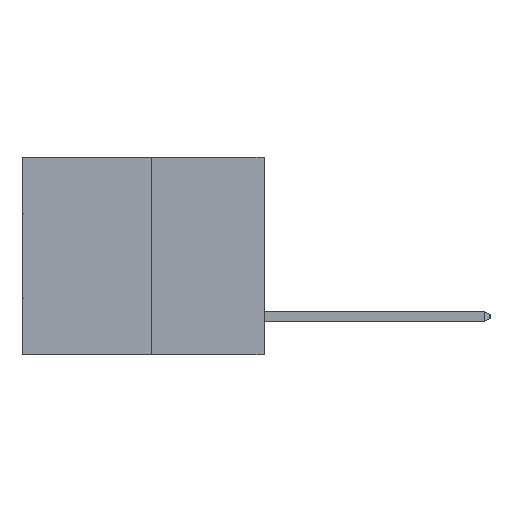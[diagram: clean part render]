
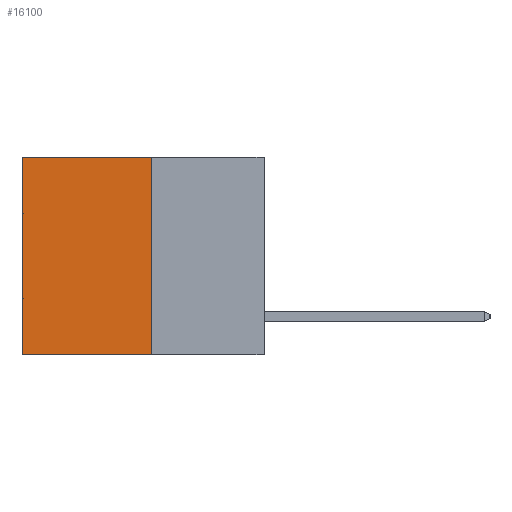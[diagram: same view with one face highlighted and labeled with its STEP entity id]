
A CAD part, left-side view. The second image highlights one B-rep face of the part: STEP entity #16100.
In plain terms, the highlighted planar face has unit normal (-1, 0, 0).
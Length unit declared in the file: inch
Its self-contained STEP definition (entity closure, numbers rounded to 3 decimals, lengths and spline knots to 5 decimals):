
#601 = CARTESIAN_POINT ( 'NONE',  ( 0.3165, 0.6, -0.49 ) ) ;
#1386 = CARTESIAN_POINT ( 'NONE',  ( 0.3165, 0.6, -0.49 ) ) ;
#1654 = ORIENTED_EDGE ( 'NONE', *, *, #6146, .F. ) ;
#3973 = ORIENTED_EDGE ( 'NONE', *, *, #23346, .T. ) ;
#5171 = CARTESIAN_POINT ( 'NONE',  ( 0.3165, 0.28, -0.49 ) ) ;
#5346 = DIRECTION ( 'NONE',  ( 1., 0., 0. ) ) ;
#6009 = EDGE_CURVE ( 'NONE', #11540, #22095, #23398, .T. ) ;
#6086 = CARTESIAN_POINT ( 'NONE',  ( 0.3165, 0.6, 0. ) ) ;
#6146 = EDGE_CURVE ( 'NONE', #7820, #22095, #13781, .T. ) ;
#6306 = CARTESIAN_POINT ( 'NONE',  ( 0.3165, 0.28, -0.49 ) ) ;
#7820 = VERTEX_POINT ( 'NONE', #5171 ) ;
#9064 = FACE_OUTER_BOUND ( 'NONE', #12457, .T. ) ;
#10021 = CARTESIAN_POINT ( 'NONE',  ( 0.3165, 0.28, 0. ) ) ;
#10143 = VECTOR ( 'NONE', #27080, 39.37008 ) ;
#10297 = DIRECTION ( 'NONE',  ( 0., 0., -1. ) ) ;
#11540 = VERTEX_POINT ( 'NONE', #6086 ) ;
#12457 = EDGE_LOOP ( 'NONE', ( #30422, #1654, #18782, #3973 ) ) ;
#13781 = LINE ( 'NONE', #21699, #14905 ) ;
#14905 = VECTOR ( 'NONE', #19558, 39.37008 ) ;
#16100 = ADVANCED_FACE ( 'NONE', ( #9064 ), #16846, .F. ) ;
#16790 = AXIS2_PLACEMENT_3D ( 'NONE', #24433, #5346, #24334 ) ;
#16846 = PLANE ( 'NONE',  #16790 ) ;
#16871 = VECTOR ( 'NONE', #10297, 39.37008 ) ;
#17256 = VERTEX_POINT ( 'NONE', #10021 ) ;
#18273 = VECTOR ( 'NONE', #28182, 39.37008 ) ;
#18782 = ORIENTED_EDGE ( 'NONE', *, *, #30556, .F. ) ;
#19558 = DIRECTION ( 'NONE',  ( 0., 1., 0. ) ) ;
#19794 = LINE ( 'NONE', #29363, #10143 ) ;
#21699 = CARTESIAN_POINT ( 'NONE',  ( 0.3165, 0.28, -0.49 ) ) ;
#22095 = VERTEX_POINT ( 'NONE', #601 ) ;
#23346 = EDGE_CURVE ( 'NONE', #17256, #11540, #19794, .T. ) ;
#23398 = LINE ( 'NONE', #1386, #16871 ) ;
#23636 = LINE ( 'NONE', #6306, #18273 ) ;
#24334 = DIRECTION ( 'NONE',  ( 0., 0., -1. ) ) ;
#24433 = CARTESIAN_POINT ( 'NONE',  ( 0.3165, 0.28, -0.49 ) ) ;
#27080 = DIRECTION ( 'NONE',  ( 0., 1., 0. ) ) ;
#28182 = DIRECTION ( 'NONE',  ( 0., 0., -1. ) ) ;
#29363 = CARTESIAN_POINT ( 'NONE',  ( 0.3165, 0.28, 0. ) ) ;
#30422 = ORIENTED_EDGE ( 'NONE', *, *, #6009, .T. ) ;
#30556 = EDGE_CURVE ( 'NONE', #17256, #7820, #23636, .T. ) ;
